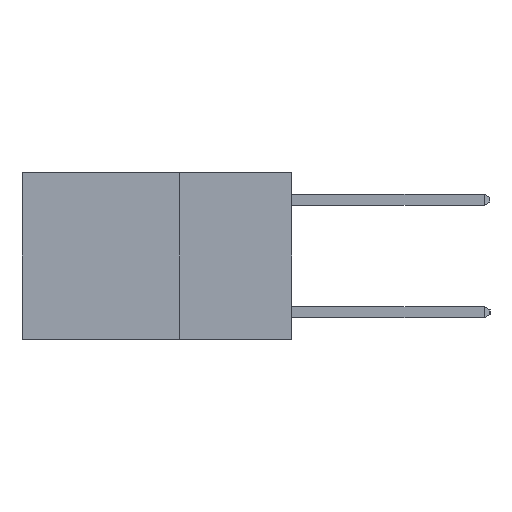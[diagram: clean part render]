
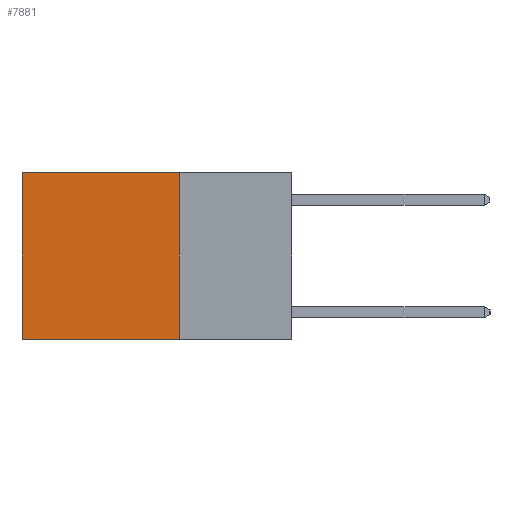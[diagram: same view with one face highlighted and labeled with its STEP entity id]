
A CAD part, left-side view. The second image highlights one B-rep face of the part: STEP entity #7881.
In plain terms, the highlighted planar face has unit normal (-1, 0, 0).
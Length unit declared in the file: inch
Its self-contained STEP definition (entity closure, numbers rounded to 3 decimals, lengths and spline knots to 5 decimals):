
#128 = CARTESIAN_POINT ( 'NONE',  ( 0.2625, 0.6, -0.37 ) ) ;
#137 = VERTEX_POINT ( 'NONE', #10124 ) ;
#534 = CARTESIAN_POINT ( 'NONE',  ( 0.2625, 0.6, 0. ) ) ;
#714 = ORIENTED_EDGE ( 'NONE', *, *, #7304, .F. ) ;
#1053 = PLANE ( 'NONE',  #11514 ) ;
#1096 = CARTESIAN_POINT ( 'NONE',  ( 0.2625, 0.25, -0.37 ) ) ;
#1110 = ORIENTED_EDGE ( 'NONE', *, *, #6869, .F. ) ;
#1328 = LINE ( 'NONE', #6509, #5958 ) ;
#1948 = VECTOR ( 'NONE', #7901, 39.37008 ) ;
#2464 = CARTESIAN_POINT ( 'NONE',  ( 0.2625, 0.25, -0.37 ) ) ;
#2965 = DIRECTION ( 'NONE',  ( 1., 0., 0. ) ) ;
#3665 = FACE_OUTER_BOUND ( 'NONE', #4976, .T. ) ;
#4367 = DIRECTION ( 'NONE',  ( 0., 1., 0. ) ) ;
#4719 = DIRECTION ( 'NONE',  ( 0., 0., -1. ) ) ;
#4882 = ORIENTED_EDGE ( 'NONE', *, *, #11680, .T. ) ;
#4976 = EDGE_LOOP ( 'NONE', ( #4882, #714, #1110, #9103 ) ) ;
#5946 = VECTOR ( 'NONE', #4367, 39.37008 ) ;
#5958 = VECTOR ( 'NONE', #4719, 39.37008 ) ;
#6064 = LINE ( 'NONE', #8037, #8397 ) ;
#6509 = CARTESIAN_POINT ( 'NONE',  ( 0.2625, 0.25, 0. ) ) ;
#6590 = CARTESIAN_POINT ( 'NONE',  ( 0.2625, 0.25, 0. ) ) ;
#6801 = LINE ( 'NONE', #534, #1948 ) ;
#6869 = EDGE_CURVE ( 'NONE', #9957, #9716, #1328, .T. ) ;
#7160 = DIRECTION ( 'NONE',  ( 0., 1., 0. ) ) ;
#7304 = EDGE_CURVE ( 'NONE', #9716, #10767, #8562, .T. ) ;
#7881 = ADVANCED_FACE ( 'NONE', ( #3665 ), #1053, .F. ) ;
#7901 = DIRECTION ( 'NONE',  ( 0., 0., -1. ) ) ;
#8037 = CARTESIAN_POINT ( 'NONE',  ( 0.2625, 0.25, 0. ) ) ;
#8329 = EDGE_CURVE ( 'NONE', #9957, #137, #6064, .T. ) ;
#8397 = VECTOR ( 'NONE', #7160, 39.37008 ) ;
#8562 = LINE ( 'NONE', #2464, #5946 ) ;
#8690 = CARTESIAN_POINT ( 'NONE',  ( 0.2625, 0.25, 0. ) ) ;
#9103 = ORIENTED_EDGE ( 'NONE', *, *, #8329, .T. ) ;
#9213 = DIRECTION ( 'NONE',  ( 0., 0., -1. ) ) ;
#9716 = VERTEX_POINT ( 'NONE', #1096 ) ;
#9957 = VERTEX_POINT ( 'NONE', #8690 ) ;
#10124 = CARTESIAN_POINT ( 'NONE',  ( 0.2625, 0.6, 0. ) ) ;
#10767 = VERTEX_POINT ( 'NONE', #128 ) ;
#11514 = AXIS2_PLACEMENT_3D ( 'NONE', #6590, #2965, #9213 ) ;
#11680 = EDGE_CURVE ( 'NONE', #137, #10767, #6801, .T. ) ;
